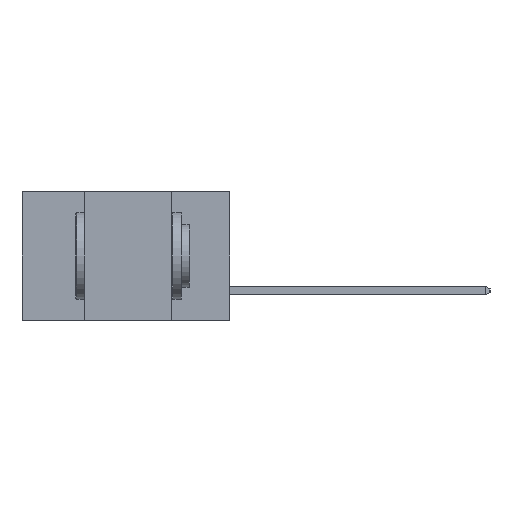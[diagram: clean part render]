
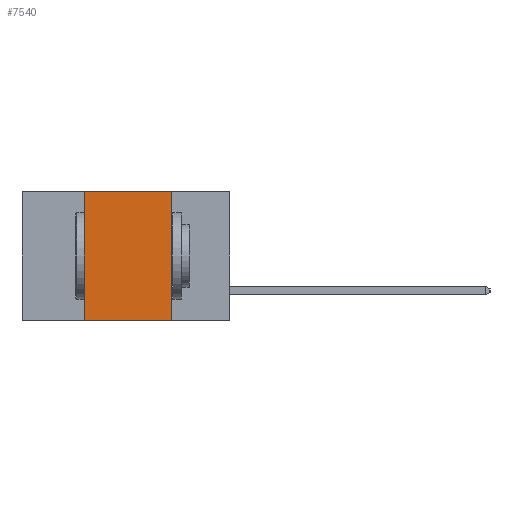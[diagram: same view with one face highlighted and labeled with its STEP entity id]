
A CAD part, left-side view. The second image highlights one B-rep face of the part: STEP entity #7540.
In plain terms, the highlighted planar face has unit normal (-1, 0, 0).
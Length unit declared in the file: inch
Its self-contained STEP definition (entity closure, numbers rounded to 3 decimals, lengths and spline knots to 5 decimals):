
#1556 = VECTOR ( 'NONE', #6487, 39.37008 ) ;
#2123 = LINE ( 'NONE', #11050, #13978 ) ;
#2266 = VERTEX_POINT ( 'NONE', #6243 ) ;
#2467 = CARTESIAN_POINT ( 'NONE',  ( 0., 0.6, -0.37 ) ) ;
#2558 = LINE ( 'NONE', #2467, #6181 ) ;
#2803 = DIRECTION ( 'NONE',  ( 0., -1., 0. ) ) ;
#3972 = EDGE_CURVE ( 'NONE', #5930, #18310, #18205, .T. ) ;
#4924 = VERTEX_POINT ( 'NONE', #9300 ) ;
#5508 = DIRECTION ( 'NONE',  ( 0., -1., 0. ) ) ;
#5930 = VERTEX_POINT ( 'NONE', #16099 ) ;
#5959 = FACE_OUTER_BOUND ( 'NONE', #12727, .T. ) ;
#6181 = VECTOR ( 'NONE', #2803, 39.37008 ) ;
#6243 = CARTESIAN_POINT ( 'NONE',  ( 0., 0.17, -0.37 ) ) ;
#6310 = CARTESIAN_POINT ( 'NONE',  ( 0., 0.42, -0.37 ) ) ;
#6487 = DIRECTION ( 'NONE',  ( 0., 0., 1. ) ) ;
#6684 = EDGE_CURVE ( 'NONE', #4924, #5930, #17865, .T. ) ;
#6910 = CARTESIAN_POINT ( 'NONE',  ( 0., 0.17, 0. ) ) ;
#7540 = ADVANCED_FACE ( 'NONE', ( #5959 ), #12551, .F. ) ;
#7728 = EDGE_CURVE ( 'NONE', #4924, #2266, #2558, .T. ) ;
#9092 = ORIENTED_EDGE ( 'NONE', *, *, #13278, .F. ) ;
#9300 = CARTESIAN_POINT ( 'NONE',  ( 0., 0.42, -0.37 ) ) ;
#9690 = ORIENTED_EDGE ( 'NONE', *, *, #7728, .T. ) ;
#9933 = CARTESIAN_POINT ( 'NONE',  ( 0., 0.6, 0. ) ) ;
#10494 = DIRECTION ( 'NONE',  ( 0., 0., -1. ) ) ;
#10514 = DIRECTION ( 'NONE',  ( 1., 0., 0. ) ) ;
#10953 = CARTESIAN_POINT ( 'NONE',  ( 0., 0.6, 0. ) ) ;
#11050 = CARTESIAN_POINT ( 'NONE',  ( 0., 0.17, -0.37 ) ) ;
#12551 = PLANE ( 'NONE',  #13164 ) ;
#12630 = DIRECTION ( 'NONE',  ( 0., 0., -1. ) ) ;
#12727 = EDGE_LOOP ( 'NONE', ( #9092, #12798, #13787, #9690 ) ) ;
#12798 = ORIENTED_EDGE ( 'NONE', *, *, #3972, .F. ) ;
#13164 = AXIS2_PLACEMENT_3D ( 'NONE', #10953, #10514, #10494 ) ;
#13278 = EDGE_CURVE ( 'NONE', #18310, #2266, #2123, .T. ) ;
#13787 = ORIENTED_EDGE ( 'NONE', *, *, #6684, .F. ) ;
#13978 = VECTOR ( 'NONE', #12630, 39.37008 ) ;
#14288 = VECTOR ( 'NONE', #5508, 39.37008 ) ;
#16099 = CARTESIAN_POINT ( 'NONE',  ( 0., 0.42, 0. ) ) ;
#17865 = LINE ( 'NONE', #6310, #1556 ) ;
#18205 = LINE ( 'NONE', #9933, #14288 ) ;
#18310 = VERTEX_POINT ( 'NONE', #6910 ) ;
